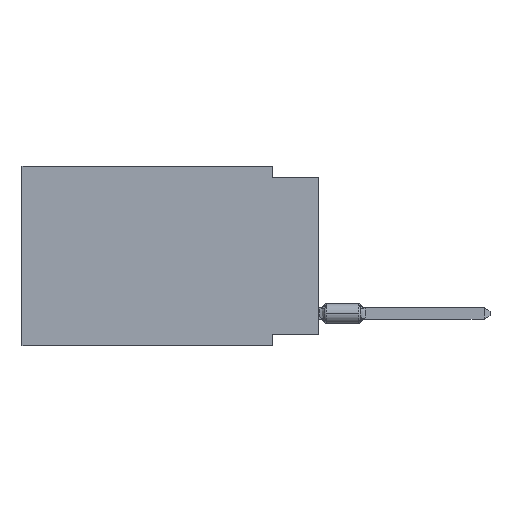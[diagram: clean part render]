
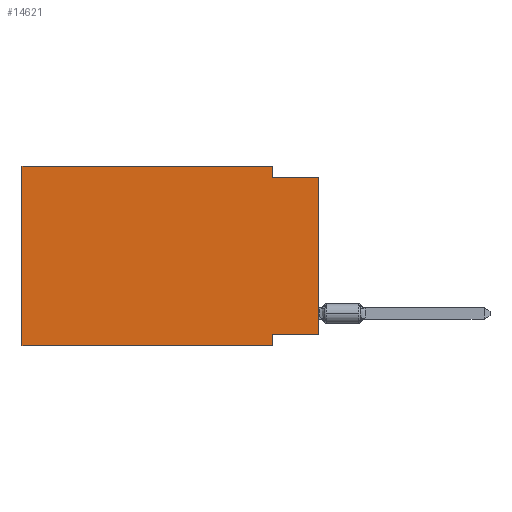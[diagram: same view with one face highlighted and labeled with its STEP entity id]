
A CAD part, left-side view. The second image highlights one B-rep face of the part: STEP entity #14621.
In plain terms, the highlighted planar face has unit normal (-1, 0, 0).
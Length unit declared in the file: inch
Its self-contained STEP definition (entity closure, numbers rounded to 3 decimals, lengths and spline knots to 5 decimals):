
#724 = EDGE_CURVE ( 'NONE', #12742, #8085, #13778, .T. ) ;
#1260 = VECTOR ( 'NONE', #14964, 39.37008 ) ;
#1419 = CARTESIAN_POINT ( 'NONE',  ( 0., 0.1, -0.365 ) ) ;
#3072 = ORIENTED_EDGE ( 'NONE', *, *, #6238, .F. ) ;
#3335 = VERTEX_POINT ( 'NONE', #4472 ) ;
#3495 = ORIENTED_EDGE ( 'NONE', *, *, #13487, .F. ) ;
#3507 = EDGE_CURVE ( 'NONE', #9428, #3811, #8453, .T. ) ;
#3558 = DIRECTION ( 'NONE',  ( 0., 0., -1. ) ) ;
#3573 = EDGE_CURVE ( 'NONE', #7092, #3335, #17173, .T. ) ;
#3811 = VERTEX_POINT ( 'NONE', #9681 ) ;
#4054 = ORIENTED_EDGE ( 'NONE', *, *, #9086, .F. ) ;
#4349 = VERTEX_POINT ( 'NONE', #15816 ) ;
#4384 = VECTOR ( 'NONE', #11567, 39.37008 ) ;
#4472 = CARTESIAN_POINT ( 'NONE',  ( 0., 0.1, -0.39 ) ) ;
#5263 = CARTESIAN_POINT ( 'NONE',  ( 0., 0., 0. ) ) ;
#5311 = CARTESIAN_POINT ( 'NONE',  ( 0., 0., -0.365 ) ) ;
#5465 = CARTESIAN_POINT ( 'NONE',  ( 0., 0.1, -0.39 ) ) ;
#6206 = DIRECTION ( 'NONE',  ( 1., 0., 0. ) ) ;
#6238 = EDGE_CURVE ( 'NONE', #8085, #3811, #6438, .T. ) ;
#6438 = LINE ( 'NONE', #7636, #7013 ) ;
#7013 = VECTOR ( 'NONE', #7732, 39.37008 ) ;
#7092 = VERTEX_POINT ( 'NONE', #1419 ) ;
#7188 = VERTEX_POINT ( 'NONE', #10461 ) ;
#7320 = PLANE ( 'NONE',  #13975 ) ;
#7591 = ORIENTED_EDGE ( 'NONE', *, *, #724, .F. ) ;
#7636 = CARTESIAN_POINT ( 'NONE',  ( 0., 0., -0.025 ) ) ;
#7732 = DIRECTION ( 'NONE',  ( 0., -1., 0. ) ) ;
#7808 = ORIENTED_EDGE ( 'NONE', *, *, #3507, .T. ) ;
#7854 = EDGE_LOOP ( 'NONE', ( #7808, #3072, #7591, #3495, #4054, #16513, #13371, #11491 ) ) ;
#8085 = VERTEX_POINT ( 'NONE', #14078 ) ;
#8453 = LINE ( 'NONE', #5263, #12740 ) ;
#8805 = FACE_OUTER_BOUND ( 'NONE', #7854, .T. ) ;
#9086 = EDGE_CURVE ( 'NONE', #4349, #7188, #17781, .T. ) ;
#9389 = VECTOR ( 'NONE', #15793, 39.37008 ) ;
#9428 = VERTEX_POINT ( 'NONE', #17757 ) ;
#9633 = LINE ( 'NONE', #15590, #9389 ) ;
#9681 = CARTESIAN_POINT ( 'NONE',  ( 0., 0., -0.025 ) ) ;
#10139 = DIRECTION ( 'NONE',  ( 0., 0., 1. ) ) ;
#10294 = CARTESIAN_POINT ( 'NONE',  ( 0., 0.645, 0. ) ) ;
#10461 = CARTESIAN_POINT ( 'NONE',  ( 0., 0.645, 0. ) ) ;
#10585 = VECTOR ( 'NONE', #10139, 39.37008 ) ;
#11199 = CARTESIAN_POINT ( 'NONE',  ( 0., 0.1, 0. ) ) ;
#11491 = ORIENTED_EDGE ( 'NONE', *, *, #17824, .F. ) ;
#11567 = DIRECTION ( 'NONE',  ( 0., 1., 0. ) ) ;
#12413 = VECTOR ( 'NONE', #18969, 39.37008 ) ;
#12740 = VECTOR ( 'NONE', #14292, 39.37008 ) ;
#12742 = VERTEX_POINT ( 'NONE', #19402 ) ;
#13110 = VECTOR ( 'NONE', #3558, 39.37008 ) ;
#13371 = ORIENTED_EDGE ( 'NONE', *, *, #3573, .F. ) ;
#13487 = EDGE_CURVE ( 'NONE', #7188, #12742, #9633, .T. ) ;
#13778 = LINE ( 'NONE', #11199, #13110 ) ;
#13975 = AXIS2_PLACEMENT_3D ( 'NONE', #10294, #6206, #14858 ) ;
#14078 = CARTESIAN_POINT ( 'NONE',  ( 0., 0.1, -0.025 ) ) ;
#14292 = DIRECTION ( 'NONE',  ( 0., 0., 1. ) ) ;
#14621 = ADVANCED_FACE ( 'NONE', ( #8805 ), #7320, .F. ) ;
#14858 = DIRECTION ( 'NONE',  ( 0., 0., -1. ) ) ;
#14863 = CARTESIAN_POINT ( 'NONE',  ( 0., 0.645, -0.39 ) ) ;
#14964 = DIRECTION ( 'NONE',  ( 0., -1., 0. ) ) ;
#15590 = CARTESIAN_POINT ( 'NONE',  ( 0., 0.645, 0. ) ) ;
#15793 = DIRECTION ( 'NONE',  ( 0., -1., 0. ) ) ;
#15816 = CARTESIAN_POINT ( 'NONE',  ( 0., 0.645, -0.39 ) ) ;
#15837 = LINE ( 'NONE', #5311, #4384 ) ;
#15875 = EDGE_CURVE ( 'NONE', #4349, #3335, #18043, .T. ) ;
#16513 = ORIENTED_EDGE ( 'NONE', *, *, #15875, .T. ) ;
#17173 = LINE ( 'NONE', #5465, #12413 ) ;
#17757 = CARTESIAN_POINT ( 'NONE',  ( 0., 0., -0.365 ) ) ;
#17781 = LINE ( 'NONE', #19559, #10585 ) ;
#17824 = EDGE_CURVE ( 'NONE', #9428, #7092, #15837, .T. ) ;
#18043 = LINE ( 'NONE', #14863, #1260 ) ;
#18969 = DIRECTION ( 'NONE',  ( 0., 0., -1. ) ) ;
#19402 = CARTESIAN_POINT ( 'NONE',  ( 0., 0.1, 0. ) ) ;
#19559 = CARTESIAN_POINT ( 'NONE',  ( 0., 0.645, 0. ) ) ;
